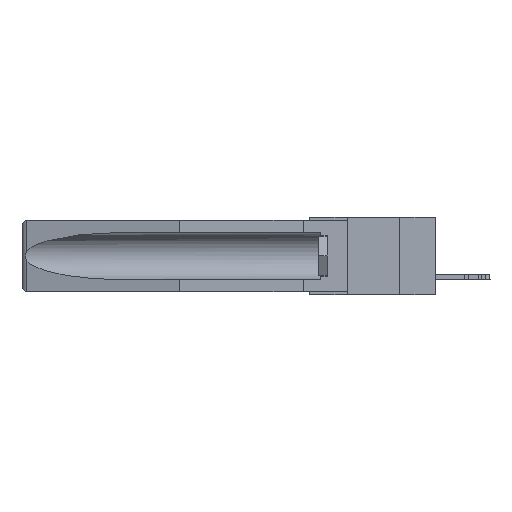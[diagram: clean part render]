
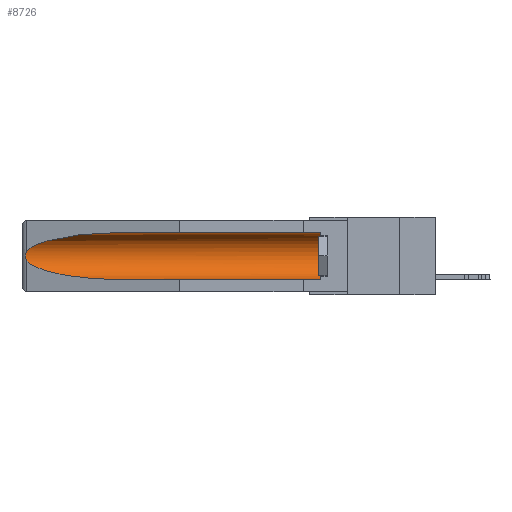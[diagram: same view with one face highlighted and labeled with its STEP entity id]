
A CAD part, left-side view. The second image highlights one B-rep face of the part: STEP entity #8726.
In plain terms, the highlighted cylindrical face has radius 2.857 mm (diameter 5.715 mm), a partial arc.
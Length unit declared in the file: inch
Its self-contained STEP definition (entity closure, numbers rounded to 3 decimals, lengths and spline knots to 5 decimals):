
#2237 = CARTESIAN_POINT ( 'NONE',  ( 0.2673, 1.5327, -0.16383 ) ) ;
#2555 = EDGE_CURVE ( 'NONE', #15247, #15547, #20260, .T. ) ;
#2767 = CARTESIAN_POINT ( 'NONE',  ( 0.155, 1.07973, -0.284 ) ) ;
#3389 = DIRECTION ( 'NONE',  ( 0., 0., 1. ) ) ;
#3768 = ORIENTED_EDGE ( 'NONE', *, *, #7284, .T. ) ;
#4495 = CARTESIAN_POINT ( 'NONE',  ( 0.2675, 1.53308, -0.16763 ) ) ;
#4689 = CARTESIAN_POINT ( 'NONE',  ( 0.21114, 1.30732, -0.059 ) ) ;
#6459 = CARTESIAN_POINT ( 'NONE',  ( 0.155, 0.126, -0.284 ) ) ;
#7142 = CARTESIAN_POINT ( 'NONE',  ( 0.155, -0.30754, -0.059 ) ) ;
#7284 = EDGE_CURVE ( 'NONE', #21728, #7446, #18327, .T. ) ;
#7446 = VERTEX_POINT ( 'NONE', #23321 ) ;
#7516 = CARTESIAN_POINT ( 'NONE',  ( 0.21114, 1.30732, -0.284 ) ) ;
#7931 = EDGE_CURVE ( 'NONE', #23809, #21728, #18172, .T. ) ;
#8500 = AXIS2_PLACEMENT_3D ( 'NONE', #19060, #16839, #3389 ) ;
#8505 = CIRCLE ( 'NONE', #14896, 0.1125 ) ;
#8576 = CARTESIAN_POINT ( 'NONE',  ( 0.2673, 1.53269, -0.17917 ) ) ;
#8677 = CARTESIAN_POINT ( 'NONE',  ( 0.26655, 1.53094, -0.18657 ) ) ;
#8726 = ADVANCED_FACE ( 'NONE', ( #24444 ), #16609, .F. ) ;
#9272 = CARTESIAN_POINT ( 'NONE',  ( 0.155, 1.07973, -0.059 ) ) ;
#10932 = CARTESIAN_POINT ( 'NONE',  ( 0.26537, 1.52718, -0.19328 ) ) ;
#11113 = CARTESIAN_POINT ( 'NONE',  ( 0.26597, 1.52961, -0.15275 ) ) ;
#11268 = CARTESIAN_POINT ( 'NONE',  ( 0.25451, 1.48313, -0.24835 ) ) ;
#11385 = CARTESIAN_POINT ( 'NONE',  ( 0.26537, 1.52718, -0.19328 ) ) ;
#11779 = EDGE_CURVE ( 'NONE', #14139, #15547, #20127, .T. ) ;
#13085 = CARTESIAN_POINT ( 'NONE',  ( 0.26537, 1.52718, -0.14972 ) ) ;
#13384 = CARTESIAN_POINT ( 'NONE',  ( 0.26654, 1.53092, -0.15636 ) ) ;
#14139 = VERTEX_POINT ( 'NONE', #11385 ) ;
#14896 = AXIS2_PLACEMENT_3D ( 'NONE', #27039, #20049, #20147 ) ;
#15247 = VERTEX_POINT ( 'NONE', #6459 ) ;
#15547 = VERTEX_POINT ( 'NONE', #16265 ) ;
#15921 = DIRECTION ( 'NONE',  ( 0., 1., 0. ) ) ;
#15961 = CARTESIAN_POINT ( 'NONE',  ( 0.25451, 1.48313, -0.09465 ) ) ;
#16265 = CARTESIAN_POINT ( 'NONE',  ( 0.155, 1.07973, -0.284 ) ) ;
#16481 = CARTESIAN_POINT ( 'NONE',  ( 0.155, -0.30754, -0.284 ) ) ;
#16609 = CYLINDRICAL_SURFACE ( 'NONE', #8500, 0.1125 ) ;
#16839 = DIRECTION ( 'NONE',  ( 0., 1., 0. ) ) ;
#17006 = B_SPLINE_CURVE_WITH_KNOTS ( 'NONE', 3,
 ( #13085, #11113, #13384, #2237, #4495, #18093, #8576, #8677, #24549, #10932 ),
 .UNSPECIFIED., .F., .F.,
 ( 4, 2, 2, 2, 4 ),
 ( 0., 0.00029, 0.00058, 0.00087, 0.00117 ),
 .UNSPECIFIED. ) ;
#17857 = EDGE_CURVE ( 'NONE', #15247, #23809, #8505, .T. ) ;
#18093 = CARTESIAN_POINT ( 'NONE',  ( 0.2675, 1.53308, -0.17534 ) ) ;
#18172 = LINE ( 'NONE', #7142, #21020 ) ;
#18327 =( BOUNDED_CURVE ( )  B_SPLINE_CURVE ( 3, ( #9272, #4689, #15961, #23043 ),
 .UNSPECIFIED., .F., .F. ) 
 B_SPLINE_CURVE_WITH_KNOTS ( ( 4, 4 ),
 ( 4.71239, 6.08839 ),
 .UNSPECIFIED. ) 
 CURVE ( )  GEOMETRIC_REPRESENTATION_ITEM ( )  RATIONAL_B_SPLINE_CURVE ( ( 1., 0.848, 0.848, 1. ) ) 
 REPRESENTATION_ITEM ( '' )  );
#18645 = EDGE_LOOP ( 'NONE', ( #3768, #26346, #21541, #21944, #18813, #22323 ) ) ;
#18813 = ORIENTED_EDGE ( 'NONE', *, *, #17857, .T. ) ;
#19060 = CARTESIAN_POINT ( 'NONE',  ( 0.155, -0.30754, -0.1715 ) ) ;
#20049 = DIRECTION ( 'NONE',  ( 0., -1., 0. ) ) ;
#20127 =( BOUNDED_CURVE ( )  B_SPLINE_CURVE ( 3, ( #22608, #11268, #7516, #2767 ),
 .UNSPECIFIED., .F., .F. ) 
 B_SPLINE_CURVE_WITH_KNOTS ( ( 4, 4 ),
 ( 0.1948, 1.5708 ),
 .UNSPECIFIED. ) 
 CURVE ( )  GEOMETRIC_REPRESENTATION_ITEM ( )  RATIONAL_B_SPLINE_CURVE ( ( 1., 0.848, 0.848, 1. ) ) 
 REPRESENTATION_ITEM ( '' )  );
#20147 = DIRECTION ( 'NONE',  ( 0., 0., 1. ) ) ;
#20260 = LINE ( 'NONE', #16481, #20603 ) ;
#20603 = VECTOR ( 'NONE', #27781, 39.37008 ) ;
#21020 = VECTOR ( 'NONE', #15921, 39.37008 ) ;
#21541 = ORIENTED_EDGE ( 'NONE', *, *, #11779, .T. ) ;
#21728 = VERTEX_POINT ( 'NONE', #21887 ) ;
#21887 = CARTESIAN_POINT ( 'NONE',  ( 0.155, 1.07973, -0.059 ) ) ;
#21944 = ORIENTED_EDGE ( 'NONE', *, *, #2555, .F. ) ;
#22323 = ORIENTED_EDGE ( 'NONE', *, *, #7931, .T. ) ;
#22608 = CARTESIAN_POINT ( 'NONE',  ( 0.26537, 1.52718, -0.19328 ) ) ;
#22792 = CARTESIAN_POINT ( 'NONE',  ( 0.155, 0.126, -0.059 ) ) ;
#23043 = CARTESIAN_POINT ( 'NONE',  ( 0.26537, 1.52718, -0.14972 ) ) ;
#23321 = CARTESIAN_POINT ( 'NONE',  ( 0.26537, 1.52718, -0.14972 ) ) ;
#23809 = VERTEX_POINT ( 'NONE', #22792 ) ;
#24444 = FACE_OUTER_BOUND ( 'NONE', #18645, .T. ) ;
#24451 = EDGE_CURVE ( 'NONE', #7446, #14139, #17006, .T. ) ;
#24549 = CARTESIAN_POINT ( 'NONE',  ( 0.26597, 1.5296, -0.19026 ) ) ;
#26346 = ORIENTED_EDGE ( 'NONE', *, *, #24451, .T. ) ;
#27039 = CARTESIAN_POINT ( 'NONE',  ( 0.155, 0.126, -0.1715 ) ) ;
#27781 = DIRECTION ( 'NONE',  ( 0., 1., 0. ) ) ;
